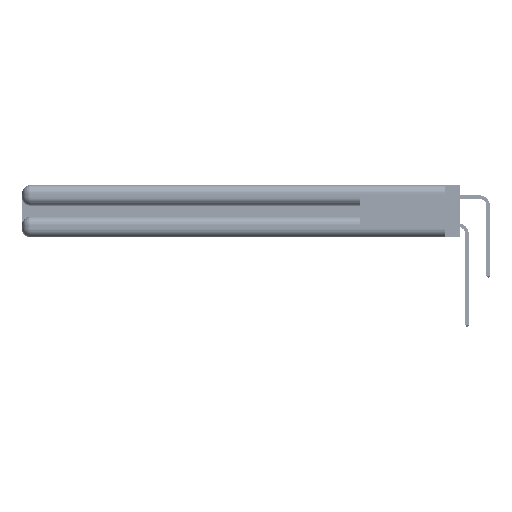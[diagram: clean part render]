
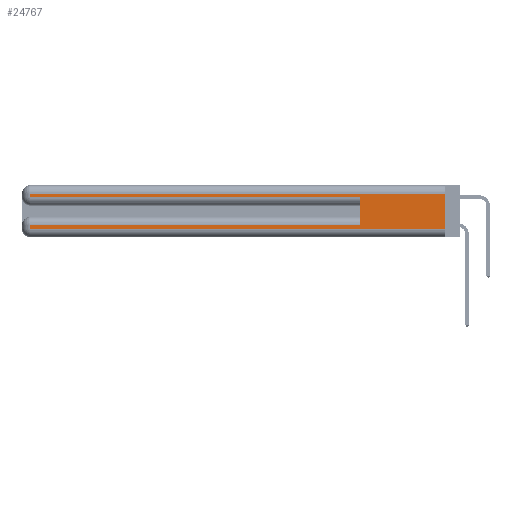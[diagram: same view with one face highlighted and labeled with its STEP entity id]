
A CAD part, left-side view. The second image highlights one B-rep face of the part: STEP entity #24767.
In plain terms, the highlighted planar face has unit normal (-1, 0, 0).
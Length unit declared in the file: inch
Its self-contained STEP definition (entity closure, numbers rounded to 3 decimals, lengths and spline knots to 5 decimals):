
#455 = EDGE_CURVE ( 'NONE', #47163, #36785, #52737, .T. ) ;
#1124 = EDGE_CURVE ( 'NONE', #14833, #9067, #43568, .T. ) ;
#1977 = CARTESIAN_POINT ( 'NONE',  ( 0., 0., 0.06 ) ) ;
#2635 = CARTESIAN_POINT ( 'NONE',  ( 0., 2.94, 0.085 ) ) ;
#2735 = ORIENTED_EDGE ( 'NONE', *, *, #1124, .T. ) ;
#5230 = CARTESIAN_POINT ( 'NONE',  ( 0., 0., 0.37 ) ) ;
#5738 = ORIENTED_EDGE ( 'NONE', *, *, #14493, .T. ) ;
#6003 = CARTESIAN_POINT ( 'NONE',  ( 0., 0.6, 0.285 ) ) ;
#7174 = CARTESIAN_POINT ( 'NONE',  ( 0., 0., 0.285 ) ) ;
#7845 = ORIENTED_EDGE ( 'NONE', *, *, #455, .F. ) ;
#8233 = VECTOR ( 'NONE', #24004, 39.37008 ) ;
#9067 = VERTEX_POINT ( 'NONE', #14901 ) ;
#9120 = CARTESIAN_POINT ( 'NONE',  ( 0., 0., 0.085 ) ) ;
#9630 = CARTESIAN_POINT ( 'NONE',  ( 0., 0.6, 0.145 ) ) ;
#10216 = VECTOR ( 'NONE', #49219, 39.37008 ) ;
#11212 = VECTOR ( 'NONE', #35077, 39.37008 ) ;
#11845 = VECTOR ( 'NONE', #33813, 39.37008 ) ;
#13838 = LINE ( 'NONE', #17154, #11845 ) ;
#14145 = EDGE_CURVE ( 'NONE', #28508, #9067, #38039, .T. ) ;
#14493 = EDGE_CURVE ( 'NONE', #16855, #36785, #27632, .T. ) ;
#14833 = VERTEX_POINT ( 'NONE', #33593 ) ;
#14901 = CARTESIAN_POINT ( 'NONE',  ( 0., 0., 0.06 ) ) ;
#15604 = EDGE_CURVE ( 'NONE', #47163, #33717, #18089, .T. ) ;
#16855 = VERTEX_POINT ( 'NONE', #50828 ) ;
#17118 = ORIENTED_EDGE ( 'NONE', *, *, #33461, .T. ) ;
#17154 = CARTESIAN_POINT ( 'NONE',  ( 0., 2.94, 0.37 ) ) ;
#17733 = EDGE_CURVE ( 'NONE', #33717, #14833, #35341, .T. ) ;
#17800 = FACE_OUTER_BOUND ( 'NONE', #41825, .T. ) ;
#18089 = LINE ( 'NONE', #9120, #35585 ) ;
#18607 = AXIS2_PLACEMENT_3D ( 'NONE', #5230, #21698, #30397 ) ;
#18692 = DIRECTION ( 'NONE',  ( 0., 0., -1. ) ) ;
#18703 = VECTOR ( 'NONE', #33794, 39.37008 ) ;
#18886 = ORIENTED_EDGE ( 'NONE', *, *, #14145, .F. ) ;
#18965 = EDGE_CURVE ( 'NONE', #44219, #16855, #13838, .T. ) ;
#21698 = DIRECTION ( 'NONE',  ( 1., 0., 0. ) ) ;
#24004 = DIRECTION ( 'NONE',  ( 0., -1., 0. ) ) ;
#24767 = ADVANCED_FACE ( 'NONE', ( #17800 ), #42495, .F. ) ;
#27632 = LINE ( 'NONE', #7174, #8233 ) ;
#28508 = VERTEX_POINT ( 'NONE', #38356 ) ;
#28869 = CARTESIAN_POINT ( 'NONE',  ( 0., 0.6, 0.085 ) ) ;
#28926 = CARTESIAN_POINT ( 'NONE',  ( 0., 0., 0.37 ) ) ;
#30397 = DIRECTION ( 'NONE',  ( 0., 0., -1. ) ) ;
#30692 = ORIENTED_EDGE ( 'NONE', *, *, #18965, .T. ) ;
#30734 = VECTOR ( 'NONE', #34979, 39.37008 ) ;
#33461 = EDGE_CURVE ( 'NONE', #28508, #44219, #40704, .T. ) ;
#33574 = DIRECTION ( 'NONE',  ( 0., 1., 0. ) ) ;
#33593 = CARTESIAN_POINT ( 'NONE',  ( 0., 2.94, 0.06 ) ) ;
#33717 = VERTEX_POINT ( 'NONE', #2635 ) ;
#33794 = DIRECTION ( 'NONE',  ( 0., 1., 0. ) ) ;
#33813 = DIRECTION ( 'NONE',  ( 0., 0., -1. ) ) ;
#34335 = CARTESIAN_POINT ( 'NONE',  ( 0., 0., 0.31 ) ) ;
#34979 = DIRECTION ( 'NONE',  ( 0., 0., 1. ) ) ;
#35077 = DIRECTION ( 'NONE',  ( 0., -1., 0. ) ) ;
#35341 = LINE ( 'NONE', #43837, #49634 ) ;
#35585 = VECTOR ( 'NONE', #33574, 39.37008 ) ;
#36785 = VERTEX_POINT ( 'NONE', #6003 ) ;
#37035 = ORIENTED_EDGE ( 'NONE', *, *, #17733, .T. ) ;
#38039 = LINE ( 'NONE', #28926, #10216 ) ;
#38356 = CARTESIAN_POINT ( 'NONE',  ( 0., 0., 0.31 ) ) ;
#40118 = CARTESIAN_POINT ( 'NONE',  ( 0., 2.94, 0.31 ) ) ;
#40704 = LINE ( 'NONE', #34335, #18703 ) ;
#41825 = EDGE_LOOP ( 'NONE', ( #18886, #17118, #30692, #5738, #7845, #45598, #37035, #2735 ) ) ;
#42495 = PLANE ( 'NONE',  #18607 ) ;
#43568 = LINE ( 'NONE', #1977, #11212 ) ;
#43837 = CARTESIAN_POINT ( 'NONE',  ( 0., 2.94, 0.37 ) ) ;
#44219 = VERTEX_POINT ( 'NONE', #40118 ) ;
#45598 = ORIENTED_EDGE ( 'NONE', *, *, #15604, .T. ) ;
#47163 = VERTEX_POINT ( 'NONE', #28869 ) ;
#49219 = DIRECTION ( 'NONE',  ( 0., 0., -1. ) ) ;
#49634 = VECTOR ( 'NONE', #18692, 39.37008 ) ;
#50828 = CARTESIAN_POINT ( 'NONE',  ( 0., 2.94, 0.285 ) ) ;
#52737 = LINE ( 'NONE', #9630, #30734 ) ;
